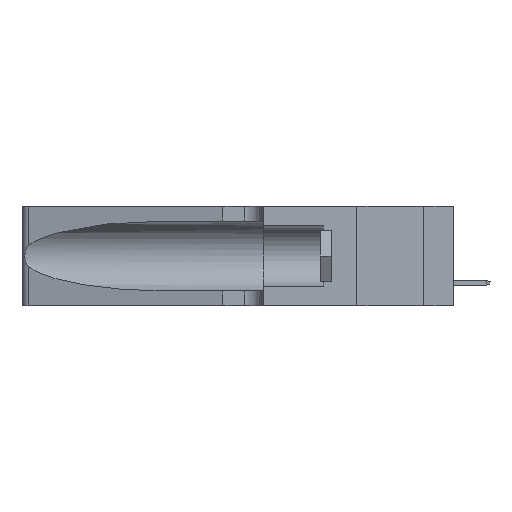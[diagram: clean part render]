
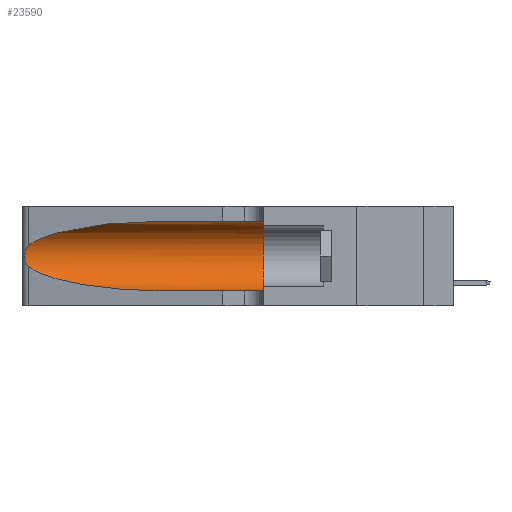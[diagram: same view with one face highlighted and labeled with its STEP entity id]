
A CAD part, left-side view. The second image highlights one B-rep face of the part: STEP entity #23590.
In plain terms, the highlighted cylindrical face has radius 3.308 mm (diameter 6.617 mm), a partial arc.
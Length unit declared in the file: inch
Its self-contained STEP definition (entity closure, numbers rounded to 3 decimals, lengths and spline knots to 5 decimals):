
#90 = ORIENTED_EDGE ( 'NONE', *, *, #25168, .F. ) ;
#345 = CARTESIAN_POINT ( 'NONE',  ( 0.25789, 1.23486, 0.15765 ) ) ;
#801 = CARTESIAN_POINT ( 'NONE',  ( 0.25639, 1.23184, 0.21858 ) ) ;
#1475 = CIRCLE ( 'NONE', #19463, 0.13025 ) ;
#1528 = LINE ( 'NONE', #20929, #30789 ) ;
#2301 = CARTESIAN_POINT ( 'NONE',  ( 0.1305, 0.72297, 0.31525 ) ) ;
#2960 = EDGE_CURVE ( 'NONE', #29159, #3397, #11967, .T. ) ;
#2966 = CARTESIAN_POINT ( 'NONE',  ( 0.26018, 1.23835, 0.19895 ) ) ;
#3397 = VERTEX_POINT ( 'NONE', #12482 ) ;
#3795 = ORIENTED_EDGE ( 'NONE', *, *, #15688, .F. ) ;
#3829 = CARTESIAN_POINT ( 'NONE',  ( 0.1305, 0.72297, 0.05475 ) ) ;
#4347 = CARTESIAN_POINT ( 'NONE',  ( 0.1305, 0.35, 0.05475 ) ) ;
#5634 = CARTESIAN_POINT ( 'NONE',  ( 0.26017, 1.23833, 0.17102 ) ) ;
#6173 = CARTESIAN_POINT ( 'NONE',  ( 0.2373, 1.15595, 0.08982 ) ) ;
#6769 = DIRECTION ( 'NONE',  ( 0., 1., 0. ) ) ;
#7182 = CARTESIAN_POINT ( 'NONE',  ( 0.1305, 1.61858, 0.185 ) ) ;
#7235 = DIRECTION ( 'NONE',  ( 0., 0., 1. ) ) ;
#7479 = VECTOR ( 'NONE', #14076, 39.37008 ) ;
#8349 = CARTESIAN_POINT ( 'NONE',  ( 0.1305, 0.35, 0.31525 ) ) ;
#9238 = CARTESIAN_POINT ( 'NONE',  ( 0.1305, 1.61858, 0.05475 ) ) ;
#9646 = VERTEX_POINT ( 'NONE', #8349 ) ;
#9723 = CARTESIAN_POINT ( 'NONE',  ( 0.25639, 1.23186, 0.15144 ) ) ;
#9864 = CARTESIAN_POINT ( 'NONE',  ( 0.25787, 1.23484, 0.2124 ) ) ;
#9976 = DIRECTION ( 'NONE',  ( 0., 0., -1. ) ) ;
#10634 = EDGE_CURVE ( 'NONE', #15367, #29159, #16313, .T. ) ;
#10642 = ORIENTED_EDGE ( 'NONE', *, *, #10634, .T. ) ;
#11258 = AXIS2_PLACEMENT_3D ( 'NONE', #7182, #12325, #9976 ) ;
#11733 = LINE ( 'NONE', #9238, #7479 ) ;
#11967 = B_SPLINE_CURVE_WITH_KNOTS ( 'NONE', 3,
 ( #27075, #19579, #801, #9864, #29419, #2966, #26615, #19887, #5634, #12518, #345, #9723, #15186, #28948 ),
 .UNSPECIFIED., .F., .F.,
 ( 4, 2, 2, 2, 2, 2, 4 ),
 ( 0., 0.00027, 0.00053, 0.00107, 0.0016, 0.00187, 0.00214 ),
 .UNSPECIFIED. ) ;
#12325 = DIRECTION ( 'NONE',  ( 0., -1., 0. ) ) ;
#12482 = CARTESIAN_POINT ( 'NONE',  ( 0.25487, 1.22718, 0.14631 ) ) ;
#12518 = CARTESIAN_POINT ( 'NONE',  ( 0.25856, 1.23593, 0.16098 ) ) ;
#12786 = EDGE_CURVE ( 'NONE', #3397, #14957, #15308, .T. ) ;
#14017 = DIRECTION ( 'NONE',  ( 0., -1., 0. ) ) ;
#14076 = DIRECTION ( 'NONE',  ( 0., -1., 0. ) ) ;
#14957 = VERTEX_POINT ( 'NONE', #25326 ) ;
#15186 = CARTESIAN_POINT ( 'NONE',  ( 0.25555, 1.22993, 0.14849 ) ) ;
#15308 =( BOUNDED_CURVE ( )  B_SPLINE_CURVE ( 3, ( #27455, #6173, #20274, #3829 ),
 .UNSPECIFIED., .F., .F. ) 
 B_SPLINE_CURVE_WITH_KNOTS ( ( 4, 4 ),
 ( 3.44316, 4.71239 ),
 .UNSPECIFIED. ) 
 CURVE ( )  GEOMETRIC_REPRESENTATION_ITEM ( )  RATIONAL_B_SPLINE_CURVE ( ( 1., 0.87, 0.87, 1. ) ) 
 REPRESENTATION_ITEM ( '' )  );
#15320 = CARTESIAN_POINT ( 'NONE',  ( 0.25487, 1.22718, 0.22369 ) ) ;
#15323 = CARTESIAN_POINT ( 'NONE',  ( 0.2373, 1.15595, 0.28018 ) ) ;
#15367 = VERTEX_POINT ( 'NONE', #2301 ) ;
#15688 = EDGE_CURVE ( 'NONE', #9646, #30878, #1475, .T. ) ;
#16114 = EDGE_CURVE ( 'NONE', #14957, #30878, #11733, .T. ) ;
#16148 = EDGE_LOOP ( 'NONE', ( #10642, #21871, #29992, #22910, #3795, #90 ) ) ;
#16313 =( BOUNDED_CURVE ( )  B_SPLINE_CURVE ( 3, ( #17369, #26905, #15323, #20348 ),
 .UNSPECIFIED., .F., .F. ) 
 B_SPLINE_CURVE_WITH_KNOTS ( ( 4, 4 ),
 ( 1.5708, 2.84003 ),
 .UNSPECIFIED. ) 
 CURVE ( )  GEOMETRIC_REPRESENTATION_ITEM ( )  RATIONAL_B_SPLINE_CURVE ( ( 1., 0.87, 0.87, 1. ) ) 
 REPRESENTATION_ITEM ( '' )  );
#17027 = FACE_OUTER_BOUND ( 'NONE', #16148, .T. ) ;
#17369 = CARTESIAN_POINT ( 'NONE',  ( 0.1305, 0.72297, 0.31525 ) ) ;
#19137 = CARTESIAN_POINT ( 'NONE',  ( 0.1305, 0.35, 0.185 ) ) ;
#19463 = AXIS2_PLACEMENT_3D ( 'NONE', #19137, #6769, #7235 ) ;
#19579 = CARTESIAN_POINT ( 'NONE',  ( 0.25555, 1.22994, 0.2215 ) ) ;
#19887 = CARTESIAN_POINT ( 'NONE',  ( 0.26075, 1.23896, 0.178 ) ) ;
#20274 = CARTESIAN_POINT ( 'NONE',  ( 0.18966, 0.96281, 0.05475 ) ) ;
#20348 = CARTESIAN_POINT ( 'NONE',  ( 0.25487, 1.22718, 0.22369 ) ) ;
#20929 = CARTESIAN_POINT ( 'NONE',  ( 0.1305, 1.61858, 0.31525 ) ) ;
#21871 = ORIENTED_EDGE ( 'NONE', *, *, #2960, .T. ) ;
#22025 = CYLINDRICAL_SURFACE ( 'NONE', #11258, 0.13025 ) ;
#22910 = ORIENTED_EDGE ( 'NONE', *, *, #16114, .T. ) ;
#23590 = ADVANCED_FACE ( 'NONE', ( #17027 ), #22025, .F. ) ;
#25168 = EDGE_CURVE ( 'NONE', #15367, #9646, #1528, .T. ) ;
#25326 = CARTESIAN_POINT ( 'NONE',  ( 0.1305, 0.72297, 0.05475 ) ) ;
#26615 = CARTESIAN_POINT ( 'NONE',  ( 0.26075, 1.23896, 0.19203 ) ) ;
#26905 = CARTESIAN_POINT ( 'NONE',  ( 0.18966, 0.96281, 0.31525 ) ) ;
#27075 = CARTESIAN_POINT ( 'NONE',  ( 0.25487, 1.22718, 0.22369 ) ) ;
#27455 = CARTESIAN_POINT ( 'NONE',  ( 0.25487, 1.22718, 0.14631 ) ) ;
#28948 = CARTESIAN_POINT ( 'NONE',  ( 0.25487, 1.22718, 0.14631 ) ) ;
#29159 = VERTEX_POINT ( 'NONE', #15320 ) ;
#29419 = CARTESIAN_POINT ( 'NONE',  ( 0.25854, 1.2359, 0.20912 ) ) ;
#29992 = ORIENTED_EDGE ( 'NONE', *, *, #12786, .T. ) ;
#30789 = VECTOR ( 'NONE', #14017, 39.37008 ) ;
#30878 = VERTEX_POINT ( 'NONE', #4347 ) ;
